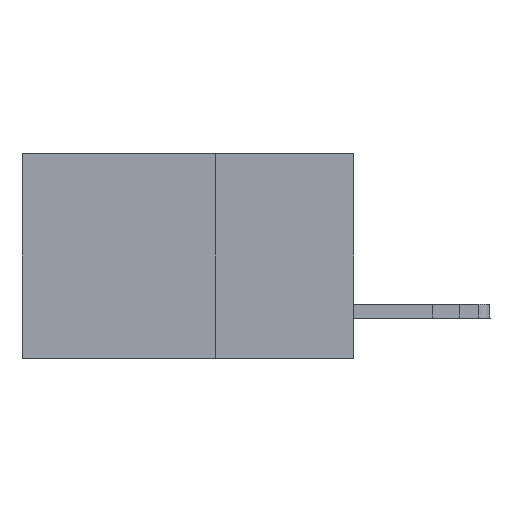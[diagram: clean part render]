
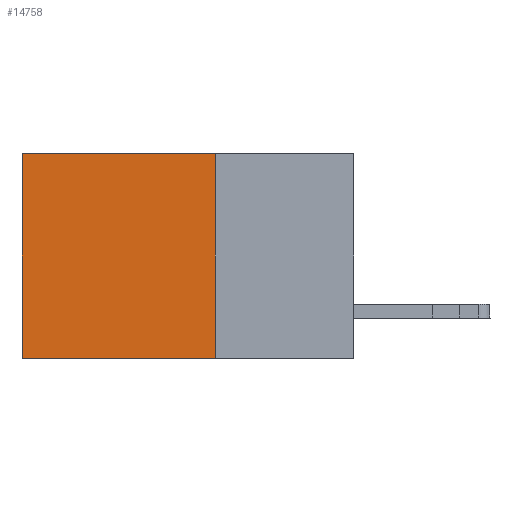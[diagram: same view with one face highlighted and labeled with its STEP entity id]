
A CAD part, left-side view. The second image highlights one B-rep face of the part: STEP entity #14758.
In plain terms, the highlighted planar face has unit normal (-1, 0, 0).
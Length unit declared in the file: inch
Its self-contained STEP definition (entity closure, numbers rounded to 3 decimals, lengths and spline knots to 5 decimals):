
#58 = CARTESIAN_POINT ( 'NONE',  ( 0.2875, 0.25, -0.37 ) ) ;
#709 = VECTOR ( 'NONE', #7986, 39.37008 ) ;
#848 = CARTESIAN_POINT ( 'NONE',  ( 0.2875, 0.25, 0. ) ) ;
#2110 = LINE ( 'NONE', #8795, #2508 ) ;
#2116 = DIRECTION ( 'NONE',  ( 0., 0., -1. ) ) ;
#2430 = ORIENTED_EDGE ( 'NONE', *, *, #12663, .T. ) ;
#2484 = CARTESIAN_POINT ( 'NONE',  ( 0.2875, 0.25, 0. ) ) ;
#2508 = VECTOR ( 'NONE', #13269, 39.37008 ) ;
#2679 = CARTESIAN_POINT ( 'NONE',  ( 0.2875, 0.6, 0. ) ) ;
#2681 = VECTOR ( 'NONE', #3213, 39.37008 ) ;
#2730 = EDGE_CURVE ( 'NONE', #10754, #12541, #5634, .T. ) ;
#2735 = VERTEX_POINT ( 'NONE', #2484 ) ;
#3213 = DIRECTION ( 'NONE',  ( 0., 0., -1. ) ) ;
#3259 = ORIENTED_EDGE ( 'NONE', *, *, #12408, .F. ) ;
#4742 = DIRECTION ( 'NONE',  ( 0., 1., 0. ) ) ;
#5634 = LINE ( 'NONE', #2679, #2681 ) ;
#5877 = CARTESIAN_POINT ( 'NONE',  ( 0.2875, 0.6, 0. ) ) ;
#6004 = ORIENTED_EDGE ( 'NONE', *, *, #2730, .T. ) ;
#6185 = EDGE_LOOP ( 'NONE', ( #6004, #3259, #6420, #2430 ) ) ;
#6420 = ORIENTED_EDGE ( 'NONE', *, *, #6582, .F. ) ;
#6582 = EDGE_CURVE ( 'NONE', #2735, #14368, #11131, .T. ) ;
#7934 = CARTESIAN_POINT ( 'NONE',  ( 0.2875, 0.25, 0. ) ) ;
#7986 = DIRECTION ( 'NONE',  ( 0., 0., -1. ) ) ;
#8300 = PLANE ( 'NONE',  #11688 ) ;
#8795 = CARTESIAN_POINT ( 'NONE',  ( 0.2875, 0.25, 0. ) ) ;
#9217 = VECTOR ( 'NONE', #4742, 39.37008 ) ;
#9438 = DIRECTION ( 'NONE',  ( 1., 0., 0. ) ) ;
#10754 = VERTEX_POINT ( 'NONE', #5877 ) ;
#10836 = CARTESIAN_POINT ( 'NONE',  ( 0.2875, 0.6, -0.37 ) ) ;
#11131 = LINE ( 'NONE', #7934, #709 ) ;
#11688 = AXIS2_PLACEMENT_3D ( 'NONE', #848, #9438, #2116 ) ;
#11759 = CARTESIAN_POINT ( 'NONE',  ( 0.2875, 0.25, -0.37 ) ) ;
#11944 = FACE_OUTER_BOUND ( 'NONE', #6185, .T. ) ;
#12199 = LINE ( 'NONE', #11759, #9217 ) ;
#12408 = EDGE_CURVE ( 'NONE', #14368, #12541, #12199, .T. ) ;
#12541 = VERTEX_POINT ( 'NONE', #10836 ) ;
#12663 = EDGE_CURVE ( 'NONE', #2735, #10754, #2110, .T. ) ;
#13269 = DIRECTION ( 'NONE',  ( 0., 1., 0. ) ) ;
#14368 = VERTEX_POINT ( 'NONE', #58 ) ;
#14758 = ADVANCED_FACE ( 'NONE', ( #11944 ), #8300, .F. ) ;
